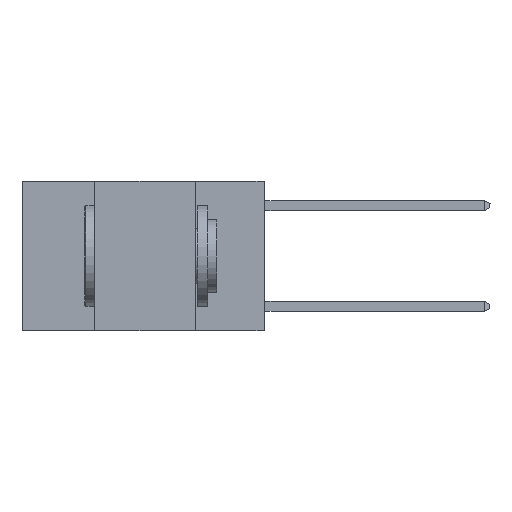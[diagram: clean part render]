
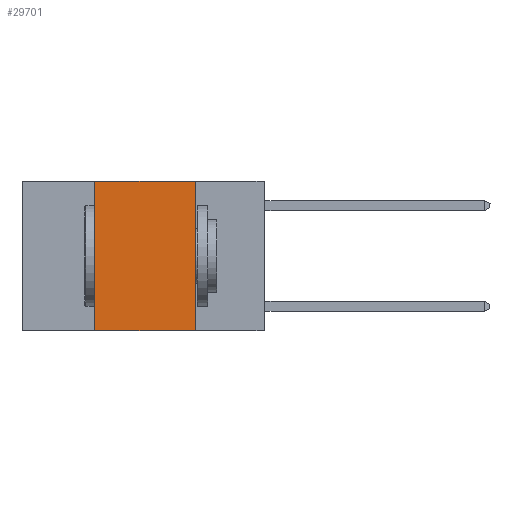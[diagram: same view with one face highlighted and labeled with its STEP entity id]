
A CAD part, left-side view. The second image highlights one B-rep face of the part: STEP entity #29701.
In plain terms, the highlighted planar face has unit normal (-1, 0, 0).
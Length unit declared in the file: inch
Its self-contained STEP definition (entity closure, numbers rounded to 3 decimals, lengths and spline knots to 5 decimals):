
#445 = EDGE_CURVE ( 'NONE', #25709, #29380, #25647, .T. ) ;
#558 = VECTOR ( 'NONE', #12841, 39.37008 ) ;
#1970 = EDGE_CURVE ( 'NONE', #29380, #23213, #27908, .T. ) ;
#4316 = CARTESIAN_POINT ( 'NONE',  ( 0., 0.17, 0. ) ) ;
#9290 = ORIENTED_EDGE ( 'NONE', *, *, #26227, .T. ) ;
#10149 = LINE ( 'NONE', #14580, #20562 ) ;
#12429 = ORIENTED_EDGE ( 'NONE', *, *, #31005, .F. ) ;
#12841 = DIRECTION ( 'NONE',  ( 0., -1., 0. ) ) ;
#13274 = FACE_OUTER_BOUND ( 'NONE', #21193, .T. ) ;
#13461 = VECTOR ( 'NONE', #16034, 39.37008 ) ;
#13609 = CARTESIAN_POINT ( 'NONE',  ( 0., 0.42, 0. ) ) ;
#13913 = LINE ( 'NONE', #13609, #22292 ) ;
#13983 = ORIENTED_EDGE ( 'NONE', *, *, #445, .F. ) ;
#14580 = CARTESIAN_POINT ( 'NONE',  ( 0., 0.6, -0.37 ) ) ;
#16034 = DIRECTION ( 'NONE',  ( 0., 0., -1. ) ) ;
#17453 = CARTESIAN_POINT ( 'NONE',  ( 0., 0.17, -0.37 ) ) ;
#18022 = CARTESIAN_POINT ( 'NONE',  ( 0., 0.6, 0. ) ) ;
#19632 = VERTEX_POINT ( 'NONE', #21612 ) ;
#19805 = DIRECTION ( 'NONE',  ( 0., -1., 0. ) ) ;
#20562 = VECTOR ( 'NONE', #19805, 39.37008 ) ;
#20569 = DIRECTION ( 'NONE',  ( 0., 0., 1. ) ) ;
#21193 = EDGE_LOOP ( 'NONE', ( #30745, #13983, #12429, #9290 ) ) ;
#21612 = CARTESIAN_POINT ( 'NONE',  ( 0., 0.42, -0.37 ) ) ;
#22292 = VECTOR ( 'NONE', #20569, 39.37008 ) ;
#23213 = VERTEX_POINT ( 'NONE', #17453 ) ;
#23394 = DIRECTION ( 'NONE',  ( 1., 0., 0. ) ) ;
#25647 = LINE ( 'NONE', #27407, #558 ) ;
#25709 = VERTEX_POINT ( 'NONE', #26487 ) ;
#25774 = PLANE ( 'NONE',  #27286 ) ;
#26227 = EDGE_CURVE ( 'NONE', #19632, #23213, #10149, .T. ) ;
#26487 = CARTESIAN_POINT ( 'NONE',  ( 0., 0.42, 0. ) ) ;
#27286 = AXIS2_PLACEMENT_3D ( 'NONE', #18022, #23394, #28150 ) ;
#27407 = CARTESIAN_POINT ( 'NONE',  ( 0., 0.6, 0. ) ) ;
#27908 = LINE ( 'NONE', #4316, #13461 ) ;
#28150 = DIRECTION ( 'NONE',  ( 0., 0., -1. ) ) ;
#29380 = VERTEX_POINT ( 'NONE', #30882 ) ;
#29701 = ADVANCED_FACE ( 'NONE', ( #13274 ), #25774, .F. ) ;
#30745 = ORIENTED_EDGE ( 'NONE', *, *, #1970, .F. ) ;
#30882 = CARTESIAN_POINT ( 'NONE',  ( 0., 0.17, 0. ) ) ;
#31005 = EDGE_CURVE ( 'NONE', #19632, #25709, #13913, .T. ) ;
